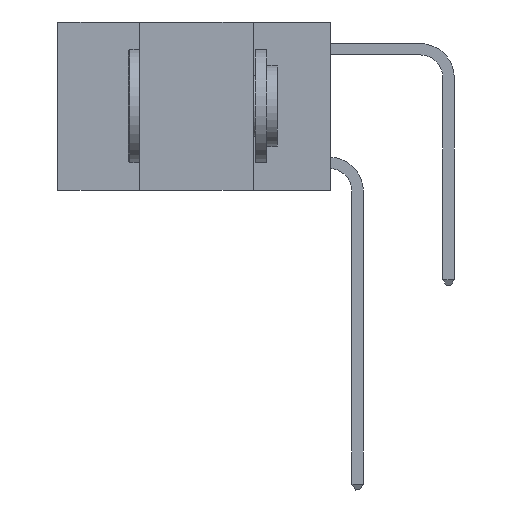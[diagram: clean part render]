
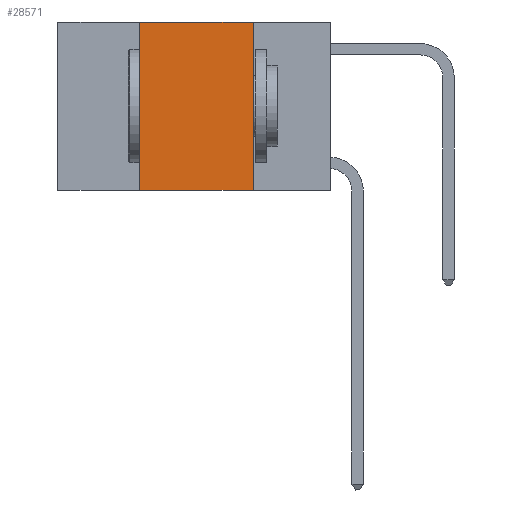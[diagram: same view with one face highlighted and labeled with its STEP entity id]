
A CAD part, left-side view. The second image highlights one B-rep face of the part: STEP entity #28571.
In plain terms, the highlighted planar face has unit normal (-1, 0, 0).
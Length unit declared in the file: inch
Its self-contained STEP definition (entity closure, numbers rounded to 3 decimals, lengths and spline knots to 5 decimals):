
#500 = EDGE_CURVE ( 'NONE', #1891, #16021, #19052, .T. ) ;
#1594 = FACE_OUTER_BOUND ( 'NONE', #24703, .T. ) ;
#1891 = VERTEX_POINT ( 'NONE', #26535 ) ;
#2317 = ORIENTED_EDGE ( 'NONE', *, *, #28850, .F. ) ;
#2441 = CARTESIAN_POINT ( 'NONE',  ( 0., 0.6, 0. ) ) ;
#3528 = DIRECTION ( 'NONE',  ( 0., -1., 0. ) ) ;
#4293 = DIRECTION ( 'NONE',  ( 0., 0., -1. ) ) ;
#4897 = DIRECTION ( 'NONE',  ( 0., 0., 1. ) ) ;
#5321 = VECTOR ( 'NONE', #4293, 39.37008 ) ;
#7445 = CARTESIAN_POINT ( 'NONE',  ( 0., 0.6, 0. ) ) ;
#7554 = DIRECTION ( 'NONE',  ( 1., 0., 0. ) ) ;
#8274 = DIRECTION ( 'NONE',  ( 0., -1., 0. ) ) ;
#8695 = ORIENTED_EDGE ( 'NONE', *, *, #500, .F. ) ;
#9719 = VECTOR ( 'NONE', #4897, 39.37008 ) ;
#10051 = CARTESIAN_POINT ( 'NONE',  ( 0., 0.42, -0.37 ) ) ;
#10195 = ORIENTED_EDGE ( 'NONE', *, *, #20827, .F. ) ;
#12419 = CARTESIAN_POINT ( 'NONE',  ( 0., 0.17, 0. ) ) ;
#13045 = CARTESIAN_POINT ( 'NONE',  ( 0., 0.6, -0.37 ) ) ;
#13578 = AXIS2_PLACEMENT_3D ( 'NONE', #7445, #7554, #24390 ) ;
#14860 = VERTEX_POINT ( 'NONE', #24597 ) ;
#16021 = VERTEX_POINT ( 'NONE', #12419 ) ;
#16619 = ORIENTED_EDGE ( 'NONE', *, *, #28640, .T. ) ;
#18125 = LINE ( 'NONE', #30469, #5321 ) ;
#19052 = LINE ( 'NONE', #2441, #23950 ) ;
#19539 = PLANE ( 'NONE',  #13578 ) ;
#20256 = VERTEX_POINT ( 'NONE', #10051 ) ;
#20827 = EDGE_CURVE ( 'NONE', #20256, #1891, #20976, .T. ) ;
#20976 = LINE ( 'NONE', #26433, #9719 ) ;
#23950 = VECTOR ( 'NONE', #3528, 39.37008 ) ;
#24175 = VECTOR ( 'NONE', #8274, 39.37008 ) ;
#24390 = DIRECTION ( 'NONE',  ( 0., 0., -1. ) ) ;
#24597 = CARTESIAN_POINT ( 'NONE',  ( 0., 0.17, -0.37 ) ) ;
#24703 = EDGE_LOOP ( 'NONE', ( #2317, #8695, #10195, #16619 ) ) ;
#26433 = CARTESIAN_POINT ( 'NONE',  ( 0., 0.42, 0. ) ) ;
#26535 = CARTESIAN_POINT ( 'NONE',  ( 0., 0.42, 0. ) ) ;
#28571 = ADVANCED_FACE ( 'NONE', ( #1594 ), #19539, .F. ) ;
#28640 = EDGE_CURVE ( 'NONE', #20256, #14860, #30448, .T. ) ;
#28850 = EDGE_CURVE ( 'NONE', #16021, #14860, #18125, .T. ) ;
#30448 = LINE ( 'NONE', #13045, #24175 ) ;
#30469 = CARTESIAN_POINT ( 'NONE',  ( 0., 0.17, 0. ) ) ;
